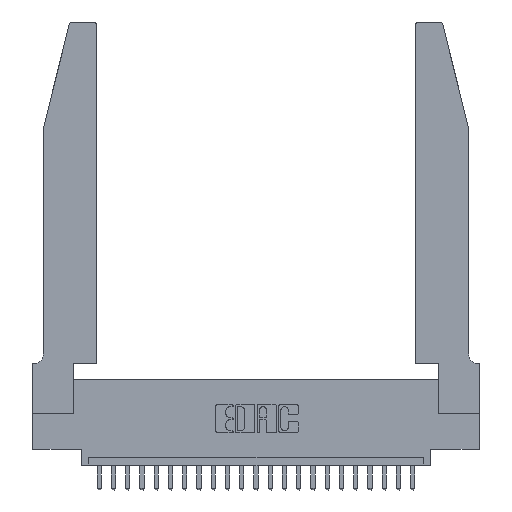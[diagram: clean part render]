
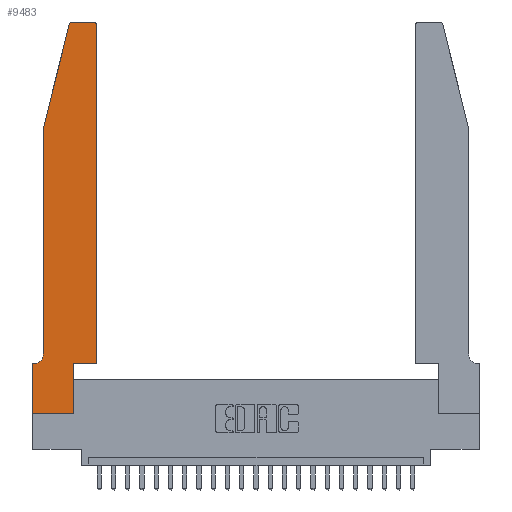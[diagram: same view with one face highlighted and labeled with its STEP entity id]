
A CAD part, top view. The second image highlights one B-rep face of the part: STEP entity #9483.
In plain terms, the highlighted planar face has unit normal (0, 0, 1).
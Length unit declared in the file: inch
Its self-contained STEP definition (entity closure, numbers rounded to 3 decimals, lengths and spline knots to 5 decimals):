
#596 = EDGE_CURVE ( 'NONE', #1482, #24212, #6929, .T. ) ;
#894 = VERTEX_POINT ( 'NONE', #23099 ) ;
#1099 = CARTESIAN_POINT ( 'NONE',  ( 0.2605, 2.75, 0.37 ) ) ;
#1107 = CARTESIAN_POINT ( 'NONE',  ( 0.4505, 0.35, 0.37 ) ) ;
#1202 = DIRECTION ( 'NONE',  ( 1., 0., 0. ) ) ;
#1482 = VERTEX_POINT ( 'NONE', #1107 ) ;
#1822 = EDGE_CURVE ( 'NONE', #22941, #23680, #2843, .T. ) ;
#2213 = VECTOR ( 'NONE', #8135, 39.37008 ) ;
#2222 = ORIENTED_EDGE ( 'NONE', *, *, #596, .T. ) ;
#2410 = DIRECTION ( 'NONE',  ( 1., 0., 0. ) ) ;
#2601 = AXIS2_PLACEMENT_3D ( 'NONE', #16537, #9131, #18574 ) ;
#2812 = CARTESIAN_POINT ( 'NONE',  ( 0.4505, 0.35, 0.37 ) ) ;
#2843 = LINE ( 'NONE', #17727, #2213 ) ;
#3376 = LINE ( 'NONE', #7257, #15073 ) ;
#3486 = CIRCLE ( 'NONE', #7518, 0.07 ) ;
#4178 = CARTESIAN_POINT ( 'NONE',  ( 0., 0., 0.37 ) ) ;
#4292 = EDGE_CURVE ( 'NONE', #894, #11102, #14121, .T. ) ;
#4366 = CIRCLE ( 'NONE', #6618, 0.03 ) ;
#4373 = ORIENTED_EDGE ( 'NONE', *, *, #4292, .T. ) ;
#4593 = VERTEX_POINT ( 'NONE', #19777 ) ;
#4614 = ORIENTED_EDGE ( 'NONE', *, *, #19599, .T. ) ;
#5080 = DIRECTION ( 'NONE',  ( -1., 0., 0. ) ) ;
#5487 = ORIENTED_EDGE ( 'NONE', *, *, #7942, .T. ) ;
#5567 = ORIENTED_EDGE ( 'NONE', *, *, #22811, .T. ) ;
#6091 = FACE_OUTER_BOUND ( 'NONE', #16807, .T. ) ;
#6618 = AXIS2_PLACEMENT_3D ( 'NONE', #7272, #22281, #1202 ) ;
#6636 = ORIENTED_EDGE ( 'NONE', *, *, #11476, .T. ) ;
#6886 = EDGE_CURVE ( 'NONE', #23680, #1482, #14878, .T. ) ;
#6921 = LINE ( 'NONE', #4178, #13195 ) ;
#6929 = LINE ( 'NONE', #2812, #8405 ) ;
#7257 = CARTESIAN_POINT ( 'NONE',  ( 0.0755, 2., 0.37 ) ) ;
#7272 = CARTESIAN_POINT ( 'NONE',  ( 0.4205, 2.72, 0.37 ) ) ;
#7518 = AXIS2_PLACEMENT_3D ( 'NONE', #22801, #18814, #16850 ) ;
#7649 = CARTESIAN_POINT ( 'NONE',  ( 0.4505, 0.35, 0.37 ) ) ;
#7942 = EDGE_CURVE ( 'NONE', #24212, #12924, #4366, .T. ) ;
#8135 = DIRECTION ( 'NONE',  ( 0., 1., 0. ) ) ;
#8208 = AXIS2_PLACEMENT_3D ( 'NONE', #24435, #12930, #22326 ) ;
#8405 = VECTOR ( 'NONE', #16336, 39.37008 ) ;
#8746 = EDGE_CURVE ( 'NONE', #18860, #18724, #3376, .T. ) ;
#8990 = VERTEX_POINT ( 'NONE', #21643 ) ;
#9077 = EDGE_CURVE ( 'NONE', #11102, #23816, #13561, .T. ) ;
#9131 = DIRECTION ( 'NONE',  ( 0., 0., 1. ) ) ;
#9483 = ADVANCED_FACE ( 'NONE', ( #6091 ), #12844, .T. ) ;
#10243 = CARTESIAN_POINT ( 'NONE',  ( 0.2865, 0., 0.37 ) ) ;
#10430 = DIRECTION ( 'NONE',  ( 0., -1., 0. ) ) ;
#10563 = ORIENTED_EDGE ( 'NONE', *, *, #18048, .T. ) ;
#10648 = CARTESIAN_POINT ( 'NONE',  ( 0.2865, 0.35, 0.37 ) ) ;
#11102 = VERTEX_POINT ( 'NONE', #24131 ) ;
#11476 = EDGE_CURVE ( 'NONE', #23816, #22941, #6921, .T. ) ;
#12844 = PLANE ( 'NONE',  #2601 ) ;
#12924 = VERTEX_POINT ( 'NONE', #21941 ) ;
#12930 = DIRECTION ( 'NONE',  ( 0., 0., 1. ) ) ;
#13195 = VECTOR ( 'NONE', #2410, 39.37008 ) ;
#13520 = VECTOR ( 'NONE', #17680, 39.37008 ) ;
#13561 = LINE ( 'NONE', #20010, #24099 ) ;
#14121 = LINE ( 'NONE', #23357, #13520 ) ;
#14196 = ORIENTED_EDGE ( 'NONE', *, *, #9077, .T. ) ;
#14878 = LINE ( 'NONE', #7649, #15766 ) ;
#15073 = VECTOR ( 'NONE', #16903, 39.37008 ) ;
#15766 = VECTOR ( 'NONE', #23082, 39.37008 ) ;
#15969 = ORIENTED_EDGE ( 'NONE', *, *, #6886, .T. ) ;
#16336 = DIRECTION ( 'NONE',  ( 0., 1., 0. ) ) ;
#16537 = CARTESIAN_POINT ( 'NONE',  ( 0., 0.35, 0.37 ) ) ;
#16778 = VECTOR ( 'NONE', #5080, 39.37008 ) ;
#16807 = EDGE_LOOP ( 'NONE', ( #10563, #5567, #17984, #19138, #4614, #4373, #14196, #6636, #22567, #15969, #2222, #5487 ) ) ;
#16850 = DIRECTION ( 'NONE',  ( -1., 0., 0. ) ) ;
#16903 = DIRECTION ( 'NONE',  ( -0.239, -0.971, 0. ) ) ;
#17462 = DIRECTION ( 'NONE',  ( 0., -1., 0. ) ) ;
#17540 = CIRCLE ( 'NONE', #8208, 0.03 ) ;
#17680 = DIRECTION ( 'NONE',  ( -1., 0., 0. ) ) ;
#17721 = CARTESIAN_POINT ( 'NONE',  ( 0.0755, 2., 0.37 ) ) ;
#17727 = CARTESIAN_POINT ( 'NONE',  ( 0.2865, 0.35, 0.37 ) ) ;
#17984 = ORIENTED_EDGE ( 'NONE', *, *, #8746, .T. ) ;
#18048 = EDGE_CURVE ( 'NONE', #12924, #8990, #20978, .T. ) ;
#18574 = DIRECTION ( 'NONE',  ( 1., 0., 0. ) ) ;
#18724 = VERTEX_POINT ( 'NONE', #22402 ) ;
#18814 = DIRECTION ( 'NONE',  ( 0., 0., -1. ) ) ;
#18860 = VERTEX_POINT ( 'NONE', #19077 ) ;
#19077 = CARTESIAN_POINT ( 'NONE',  ( 0.25487, 2.72718, 0.37 ) ) ;
#19138 = ORIENTED_EDGE ( 'NONE', *, *, #21046, .T. ) ;
#19599 = EDGE_CURVE ( 'NONE', #4593, #894, #3486, .T. ) ;
#19777 = CARTESIAN_POINT ( 'NONE',  ( 0.0755, 0.42, 0.37 ) ) ;
#19879 = VECTOR ( 'NONE', #17462, 39.37008 ) ;
#20010 = CARTESIAN_POINT ( 'NONE',  ( 0., 0., 0.37 ) ) ;
#20483 = LINE ( 'NONE', #17721, #19879 ) ;
#20978 = LINE ( 'NONE', #1099, #16778 ) ;
#21046 = EDGE_CURVE ( 'NONE', #18724, #4593, #20483, .T. ) ;
#21643 = CARTESIAN_POINT ( 'NONE',  ( 0.284, 2.75, 0.37 ) ) ;
#21941 = CARTESIAN_POINT ( 'NONE',  ( 0.4205, 2.75, 0.37 ) ) ;
#22281 = DIRECTION ( 'NONE',  ( 0., 0., 1. ) ) ;
#22326 = DIRECTION ( 'NONE',  ( 1., 0., 0. ) ) ;
#22402 = CARTESIAN_POINT ( 'NONE',  ( 0.0755, 2., 0.37 ) ) ;
#22567 = ORIENTED_EDGE ( 'NONE', *, *, #1822, .T. ) ;
#22615 = CARTESIAN_POINT ( 'NONE',  ( 0., 0., 0.37 ) ) ;
#22801 = CARTESIAN_POINT ( 'NONE',  ( 0.0055, 0.42, 0.37 ) ) ;
#22811 = EDGE_CURVE ( 'NONE', #8990, #18860, #17540, .T. ) ;
#22941 = VERTEX_POINT ( 'NONE', #10243 ) ;
#23082 = DIRECTION ( 'NONE',  ( 1., 0., 0. ) ) ;
#23099 = CARTESIAN_POINT ( 'NONE',  ( 0.0055, 0.35, 0.37 ) ) ;
#23357 = CARTESIAN_POINT ( 'NONE',  ( 0.0755, 0.35, 0.37 ) ) ;
#23680 = VERTEX_POINT ( 'NONE', #10648 ) ;
#23816 = VERTEX_POINT ( 'NONE', #22615 ) ;
#23843 = CARTESIAN_POINT ( 'NONE',  ( 0.4505, 2.72, 0.37 ) ) ;
#24099 = VECTOR ( 'NONE', #10430, 39.37008 ) ;
#24131 = CARTESIAN_POINT ( 'NONE',  ( 0., 0.35, 0.37 ) ) ;
#24212 = VERTEX_POINT ( 'NONE', #23843 ) ;
#24435 = CARTESIAN_POINT ( 'NONE',  ( 0.284, 2.72, 0.37 ) ) ;
